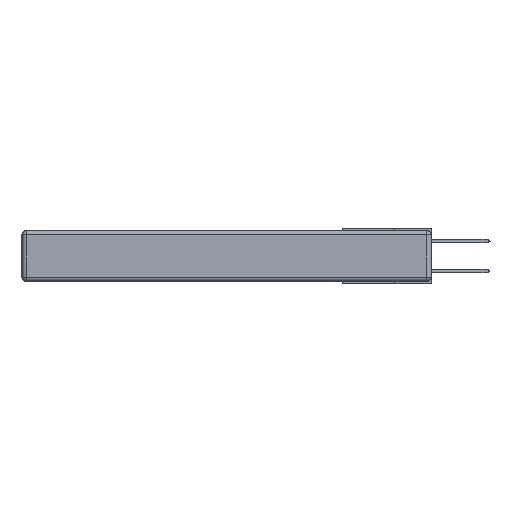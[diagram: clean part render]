
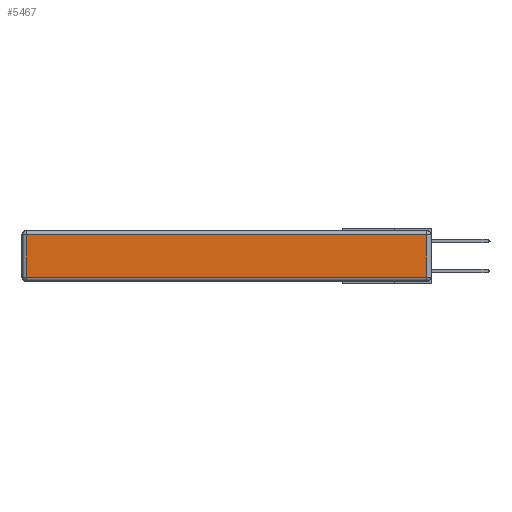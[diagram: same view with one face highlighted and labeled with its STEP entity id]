
A CAD part, left-side view. The second image highlights one B-rep face of the part: STEP entity #5467.
In plain terms, the highlighted planar face has unit normal (-1, 0, 0).
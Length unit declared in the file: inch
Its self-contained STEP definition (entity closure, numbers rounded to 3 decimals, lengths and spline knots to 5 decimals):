
#169 = ORIENTED_EDGE ( 'NONE', *, *, #16698, .T. ) ;
#472 = DIRECTION ( 'NONE',  ( 0., 1., 0. ) ) ;
#639 = PLANE ( 'NONE',  #18276 ) ;
#1341 = EDGE_CURVE ( 'NONE', #7842, #5863, #11163, .T. ) ;
#2185 = CARTESIAN_POINT ( 'NONE',  ( 0., 0.03, -0.313 ) ) ;
#3335 = EDGE_CURVE ( 'NONE', #11681, #8819, #10392, .T. ) ;
#3556 = EDGE_CURVE ( 'NONE', #8819, #7842, #10855, .T. ) ;
#3782 = CARTESIAN_POINT ( 'NONE',  ( 0., 0.03, -0.343 ) ) ;
#5467 = ADVANCED_FACE ( 'NONE', ( #10872 ), #639, .T. ) ;
#5863 = VERTEX_POINT ( 'NONE', #11854 ) ;
#6425 = VECTOR ( 'NONE', #9813, 39.37008 ) ;
#7842 = VERTEX_POINT ( 'NONE', #14080 ) ;
#7872 = DIRECTION ( 'NONE',  ( 0., 0., 1. ) ) ;
#8267 = CARTESIAN_POINT ( 'NONE',  ( 0., 0.03, -0.03 ) ) ;
#8819 = VERTEX_POINT ( 'NONE', #8267 ) ;
#9202 = LINE ( 'NONE', #17352, #6425 ) ;
#9521 = ORIENTED_EDGE ( 'NONE', *, *, #1341, .T. ) ;
#9813 = DIRECTION ( 'NONE',  ( 0., -1., 0. ) ) ;
#10392 = LINE ( 'NONE', #3782, #13879 ) ;
#10855 = LINE ( 'NONE', #12364, #14601 ) ;
#10872 = FACE_OUTER_BOUND ( 'NONE', #12662, .T. ) ;
#11163 = LINE ( 'NONE', #12551, #18638 ) ;
#11681 = VERTEX_POINT ( 'NONE', #2185 ) ;
#11771 = ORIENTED_EDGE ( 'NONE', *, *, #3556, .T. ) ;
#11854 = CARTESIAN_POINT ( 'NONE',  ( 0., 2.72, -0.313 ) ) ;
#11969 = ORIENTED_EDGE ( 'NONE', *, *, #3335, .T. ) ;
#12364 = CARTESIAN_POINT ( 'NONE',  ( 0., 2.75, -0.03 ) ) ;
#12551 = CARTESIAN_POINT ( 'NONE',  ( 0., 2.72, -0.343 ) ) ;
#12662 = EDGE_LOOP ( 'NONE', ( #169, #11969, #11771, #9521 ) ) ;
#13879 = VECTOR ( 'NONE', #16031, 39.37008 ) ;
#14056 = DIRECTION ( 'NONE',  ( 0., 0., -1. ) ) ;
#14080 = CARTESIAN_POINT ( 'NONE',  ( 0., 2.72, -0.03 ) ) ;
#14601 = VECTOR ( 'NONE', #472, 39.37008 ) ;
#15216 = CARTESIAN_POINT ( 'NONE',  ( 0., 0., -0.343 ) ) ;
#16031 = DIRECTION ( 'NONE',  ( 0., 0., 1. ) ) ;
#16698 = EDGE_CURVE ( 'NONE', #5863, #11681, #9202, .T. ) ;
#16781 = DIRECTION ( 'NONE',  ( -1., 0., 0. ) ) ;
#17352 = CARTESIAN_POINT ( 'NONE',  ( 0., 0., -0.313 ) ) ;
#18276 = AXIS2_PLACEMENT_3D ( 'NONE', #15216, #16781, #7872 ) ;
#18638 = VECTOR ( 'NONE', #14056, 39.37008 ) ;
